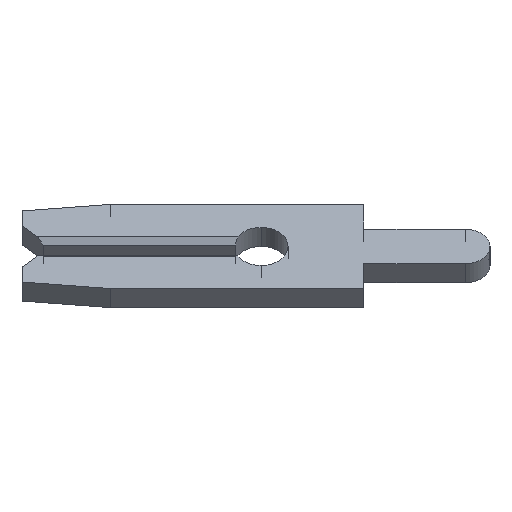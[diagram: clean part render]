
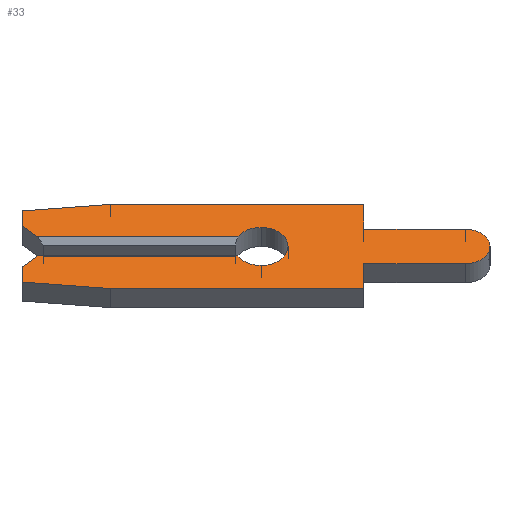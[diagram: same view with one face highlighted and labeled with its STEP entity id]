
A CAD part, left-side view. The second image highlights one B-rep face of the part: STEP entity #33.
In plain terms, the highlighted face is planar.
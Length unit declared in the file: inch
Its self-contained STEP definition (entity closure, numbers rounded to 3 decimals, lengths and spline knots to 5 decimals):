
#23 = VECTOR ( 'NONE', #1475, 39.37008 ) ;
#33 = ADVANCED_FACE ( 'NONE', ( #1533 ), #396, .F. ) ;
#50 = LINE ( 'NONE', #1919, #324 ) ;
#52 = EDGE_CURVE ( 'NONE', #813, #215, #1809, .T. ) ;
#55 = VERTEX_POINT ( 'NONE', #802 ) ;
#56 = DIRECTION ( 'NONE',  ( 0., 0., -1. ) ) ;
#65 = ORIENTED_EDGE ( 'NONE', *, *, #1874, .F. ) ;
#74 = DIRECTION ( 'NONE',  ( -1., 0., 0. ) ) ;
#77 = CARTESIAN_POINT ( 'NONE',  ( -0.013, 0.231, 0.028 ) ) ;
#80 = ORIENTED_EDGE ( 'NONE', *, *, #139, .F. ) ;
#99 = DIRECTION ( 'NONE',  ( 0., 0.707, 0.707 ) ) ;
#101 = AXIS2_PLACEMENT_3D ( 'NONE', #1152, #416, #1457 ) ;
#108 = CARTESIAN_POINT ( 'NONE',  ( -0.013, -0.099, -0.0575 ) ) ;
#135 = EDGE_LOOP ( 'NONE', ( #748, #962, #1868, #65, #1017, #488, #1345, #1728, #1633, #1066, #282, #1253, #1493, #868, #143, #161, #1041, #80 ) ) ;
#139 = EDGE_CURVE ( 'NONE', #490, #1333, #1518, .T. ) ;
#143 = ORIENTED_EDGE ( 'NONE', *, *, #636, .F. ) ;
#147 = CARTESIAN_POINT ( 'NONE',  ( -0.013, 0.216, 0.013 ) ) ;
#151 = CARTESIAN_POINT ( 'NONE',  ( -0.013, -0.1975, 0.0235 ) ) ;
#161 = ORIENTED_EDGE ( 'NONE', *, *, #1170, .F. ) ;
#167 = VERTEX_POINT ( 'NONE', #1190 ) ;
#193 = VECTOR ( 'NONE', #99, 39.37008 ) ;
#195 = EDGE_CURVE ( 'NONE', #217, #1281, #1165, .T. ) ;
#215 = VERTEX_POINT ( 'NONE', #1032 ) ;
#217 = VERTEX_POINT ( 'NONE', #151 ) ;
#219 = CARTESIAN_POINT ( 'NONE',  ( -0.013, 0.231, 0.013 ) ) ;
#241 = EDGE_CURVE ( 'NONE', #1391, #471, #313, .T. ) ;
#249 = DIRECTION ( 'NONE',  ( 0., 0., -1. ) ) ;
#277 = AXIS2_PLACEMENT_3D ( 'NONE', #1856, #1579, #56 ) ;
#282 = ORIENTED_EDGE ( 'NONE', *, *, #1658, .F. ) ;
#306 = AXIS2_PLACEMENT_3D ( 'NONE', #1734, #74, #533 ) ;
#313 = LINE ( 'NONE', #1174, #1063 ) ;
#319 = CARTESIAN_POINT ( 'NONE',  ( -0.013, 0.146, -0.0575 ) ) ;
#324 = VECTOR ( 'NONE', #1021, 39.37008 ) ;
#338 = VECTOR ( 'NONE', #987, 39.37008 ) ;
#376 = AXIS2_PLACEMENT_3D ( 'NONE', #754, #1807, #1366 ) ;
#383 = VECTOR ( 'NONE', #978, 39.37008 ) ;
#396 = PLANE ( 'NONE',  #1140 ) ;
#400 = LINE ( 'NONE', #996, #338 ) ;
#403 = LINE ( 'NONE', #1570, #892 ) ;
#416 = DIRECTION ( 'NONE',  ( 1., 0., 0. ) ) ;
#417 = EDGE_CURVE ( 'NONE', #1667, #1273, #50, .T. ) ;
#423 = VECTOR ( 'NONE', #1786, 39.37008 ) ;
#444 = EDGE_CURVE ( 'NONE', #215, #1667, #1295, .T. ) ;
#471 = VERTEX_POINT ( 'NONE', #319 ) ;
#488 = ORIENTED_EDGE ( 'NONE', *, *, #444, .F. ) ;
#490 = VERTEX_POINT ( 'NONE', #147 ) ;
#533 = DIRECTION ( 'NONE',  ( 0., 0., -1. ) ) ;
#549 = CARTESIAN_POINT ( 'NONE',  ( -0.013, 0.231, 0.04857 ) ) ;
#566 = CARTESIAN_POINT ( 'NONE',  ( -0.013, -0.099, -0.0235 ) ) ;
#571 = CARTESIAN_POINT ( 'NONE',  ( -0.013, 0.2105, -0.0075 ) ) ;
#577 = LINE ( 'NONE', #1617, #668 ) ;
#623 = LINE ( 'NONE', #1298, #1796 ) ;
#627 = CARTESIAN_POINT ( 'NONE',  ( -0.013, 0.231, -0.04857 ) ) ;
#636 = EDGE_CURVE ( 'NONE', #1688, #1930, #1747, .T. ) ;
#668 = VECTOR ( 'NONE', #1452, 39.37008 ) ;
#672 = CIRCLE ( 'NONE', #306, 0.026 ) ;
#683 = DIRECTION ( 'NONE',  ( 0., 0., 1. ) ) ;
#707 = DIRECTION ( 'NONE',  ( 0., 1., 0. ) ) ;
#716 = LINE ( 'NONE', #108, #23 ) ;
#728 = CARTESIAN_POINT ( 'NONE',  ( -0.013, 0.216, -0.013 ) ) ;
#748 = ORIENTED_EDGE ( 'NONE', *, *, #1062, .T. ) ;
#751 = DIRECTION ( 'NONE',  ( 0., -1., 0. ) ) ;
#754 = CARTESIAN_POINT ( 'NONE',  ( -0.013, 0., 0. ) ) ;
#765 = LINE ( 'NONE', #1262, #423 ) ;
#788 = LINE ( 'NONE', #1101, #1665 ) ;
#798 = CARTESIAN_POINT ( 'NONE',  ( -0.013, 0.02252, 0.013 ) ) ;
#802 = CARTESIAN_POINT ( 'NONE',  ( -0.013, -0.099, 0.0235 ) ) ;
#813 = VERTEX_POINT ( 'NONE', #627 ) ;
#828 = CARTESIAN_POINT ( 'NONE',  ( -0.013, -0.099, -0.0575 ) ) ;
#868 = ORIENTED_EDGE ( 'NONE', *, *, #1350, .F. ) ;
#872 = CARTESIAN_POINT ( 'NONE',  ( -0.013, 0.146, 0.0575 ) ) ;
#892 = VECTOR ( 'NONE', #1429, 39.37008 ) ;
#900 = CARTESIAN_POINT ( 'NONE',  ( -0.013, -0.099, 0.0575 ) ) ;
#915 = CARTESIAN_POINT ( 'NONE',  ( -0.013, 0., 0.026 ) ) ;
#954 = CARTESIAN_POINT ( 'NONE',  ( -0.013, 0.02252, -0.013 ) ) ;
#958 = VERTEX_POINT ( 'NONE', #915 ) ;
#962 = ORIENTED_EDGE ( 'NONE', *, *, #1054, .F. ) ;
#978 = DIRECTION ( 'NONE',  ( 0., -1., 0. ) ) ;
#987 = DIRECTION ( 'NONE',  ( 0., 0., 1. ) ) ;
#992 = CIRCLE ( 'NONE', #277, 0.026 ) ;
#996 = CARTESIAN_POINT ( 'NONE',  ( -0.013, 0.231, 0.028 ) ) ;
#1007 = VERTEX_POINT ( 'NONE', #798 ) ;
#1017 = ORIENTED_EDGE ( 'NONE', *, *, #417, .F. ) ;
#1021 = DIRECTION ( 'NONE',  ( 0., -1., 0. ) ) ;
#1032 = CARTESIAN_POINT ( 'NONE',  ( -0.013, 0.231, -0.028 ) ) ;
#1041 = ORIENTED_EDGE ( 'NONE', *, *, #1454, .F. ) ;
#1054 = EDGE_CURVE ( 'NONE', #958, #1007, #992, .T. ) ;
#1062 = EDGE_CURVE ( 'NONE', #490, #1007, #1212, .T. ) ;
#1063 = VECTOR ( 'NONE', #707, 39.37008 ) ;
#1066 = ORIENTED_EDGE ( 'NONE', *, *, #1775, .F. ) ;
#1101 = CARTESIAN_POINT ( 'NONE',  ( -0.013, 0.231, -0.04857 ) ) ;
#1140 = AXIS2_PLACEMENT_3D ( 'NONE', #1447, #1289, #1736 ) ;
#1152 = CARTESIAN_POINT ( 'NONE',  ( -0.013, -0.1975, 0. ) ) ;
#1165 = CIRCLE ( 'NONE', #101, 0.0235 ) ;
#1170 = EDGE_CURVE ( 'NONE', #1508, #1688, #403, .T. ) ;
#1174 = CARTESIAN_POINT ( 'NONE',  ( -0.013, 0.146, -0.0575 ) ) ;
#1190 = CARTESIAN_POINT ( 'NONE',  ( -0.013, 0., -0.026 ) ) ;
#1212 = LINE ( 'NONE', #219, #383 ) ;
#1247 = EDGE_CURVE ( 'NONE', #471, #813, #788, .T. ) ;
#1253 = ORIENTED_EDGE ( 'NONE', *, *, #195, .F. ) ;
#1262 = CARTESIAN_POINT ( 'NONE',  ( -0.013, -0.099, -0.0235 ) ) ;
#1269 = DIRECTION ( 'NONE',  ( 0., 0.995, 0.105 ) ) ;
#1273 = VERTEX_POINT ( 'NONE', #954 ) ;
#1281 = VERTEX_POINT ( 'NONE', #1583 ) ;
#1289 = DIRECTION ( 'NONE',  ( 1., 0., 0. ) ) ;
#1295 = LINE ( 'NONE', #571, #1817 ) ;
#1296 = EDGE_CURVE ( 'NONE', #167, #958, #672, .T. ) ;
#1298 = CARTESIAN_POINT ( 'NONE',  ( -0.013, -0.099, 0.0575 ) ) ;
#1333 = VERTEX_POINT ( 'NONE', #77 ) ;
#1345 = ORIENTED_EDGE ( 'NONE', *, *, #52, .F. ) ;
#1350 = EDGE_CURVE ( 'NONE', #1930, #55, #623, .T. ) ;
#1352 = VECTOR ( 'NONE', #751, 39.37008 ) ;
#1366 = DIRECTION ( 'NONE',  ( 0., 0., -1. ) ) ;
#1368 = CARTESIAN_POINT ( 'NONE',  ( -0.013, 0.146, 0.0575 ) ) ;
#1391 = VERTEX_POINT ( 'NONE', #828 ) ;
#1426 = CARTESIAN_POINT ( 'NONE',  ( -0.013, 0.231, -0.028 ) ) ;
#1429 = DIRECTION ( 'NONE',  ( 0., -0.995, 0.105 ) ) ;
#1447 = CARTESIAN_POINT ( 'NONE',  ( -0.013, 0., 0. ) ) ;
#1452 = DIRECTION ( 'NONE',  ( 0., -1., 0. ) ) ;
#1454 = EDGE_CURVE ( 'NONE', #1333, #1508, #400, .T. ) ;
#1457 = DIRECTION ( 'NONE',  ( 0., 0., 1. ) ) ;
#1475 = DIRECTION ( 'NONE',  ( 0., 0., -1. ) ) ;
#1481 = VECTOR ( 'NONE', #683, 39.37008 ) ;
#1493 = ORIENTED_EDGE ( 'NONE', *, *, #1539, .F. ) ;
#1508 = VERTEX_POINT ( 'NONE', #549 ) ;
#1518 = LINE ( 'NONE', #1763, #193 ) ;
#1533 = FACE_OUTER_BOUND ( 'NONE', #135, .T. ) ;
#1539 = EDGE_CURVE ( 'NONE', #55, #217, #577, .T. ) ;
#1570 = CARTESIAN_POINT ( 'NONE',  ( -0.013, 0.231, 0.04857 ) ) ;
#1579 = DIRECTION ( 'NONE',  ( -1., 0., 0. ) ) ;
#1583 = CARTESIAN_POINT ( 'NONE',  ( -0.013, -0.1975, -0.0235 ) ) ;
#1591 = CIRCLE ( 'NONE', #376, 0.026 ) ;
#1617 = CARTESIAN_POINT ( 'NONE',  ( -0.013, -0.099, 0.0235 ) ) ;
#1618 = VERTEX_POINT ( 'NONE', #566 ) ;
#1633 = ORIENTED_EDGE ( 'NONE', *, *, #241, .F. ) ;
#1658 = EDGE_CURVE ( 'NONE', #1281, #1618, #765, .T. ) ;
#1665 = VECTOR ( 'NONE', #1269, 39.37008 ) ;
#1667 = VERTEX_POINT ( 'NONE', #728 ) ;
#1688 = VERTEX_POINT ( 'NONE', #872 ) ;
#1728 = ORIENTED_EDGE ( 'NONE', *, *, #1247, .F. ) ;
#1734 = CARTESIAN_POINT ( 'NONE',  ( -0.013, 0., 0. ) ) ;
#1736 = DIRECTION ( 'NONE',  ( 0., 0., -1. ) ) ;
#1747 = LINE ( 'NONE', #1368, #1352 ) ;
#1763 = CARTESIAN_POINT ( 'NONE',  ( -0.013, 0.2105, 0.0075 ) ) ;
#1771 = DIRECTION ( 'NONE',  ( 0., -0.707, 0.707 ) ) ;
#1775 = EDGE_CURVE ( 'NONE', #1618, #1391, #716, .T. ) ;
#1786 = DIRECTION ( 'NONE',  ( 0., 1., 0. ) ) ;
#1796 = VECTOR ( 'NONE', #249, 39.37008 ) ;
#1807 = DIRECTION ( 'NONE',  ( -1., 0., 0. ) ) ;
#1809 = LINE ( 'NONE', #1426, #1481 ) ;
#1817 = VECTOR ( 'NONE', #1771, 39.37008 ) ;
#1856 = CARTESIAN_POINT ( 'NONE',  ( -0.013, 0., 0. ) ) ;
#1868 = ORIENTED_EDGE ( 'NONE', *, *, #1296, .F. ) ;
#1874 = EDGE_CURVE ( 'NONE', #1273, #167, #1591, .T. ) ;
#1919 = CARTESIAN_POINT ( 'NONE',  ( -0.013, 0., -0.013 ) ) ;
#1930 = VERTEX_POINT ( 'NONE', #900 ) ;
